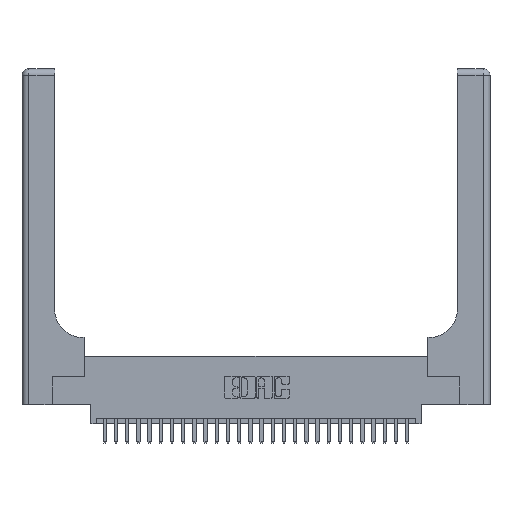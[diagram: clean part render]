
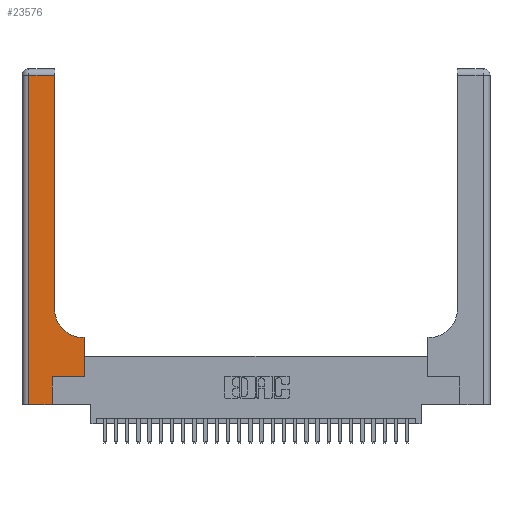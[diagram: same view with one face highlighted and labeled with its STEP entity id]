
A CAD part, top view. The second image highlights one B-rep face of the part: STEP entity #23576.
In plain terms, the highlighted planar face has unit normal (0, 0, 1).
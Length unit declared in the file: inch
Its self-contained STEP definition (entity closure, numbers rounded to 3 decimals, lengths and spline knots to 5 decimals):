
#175 = VERTEX_POINT ( 'NONE', #16787 ) ;
#555 = EDGE_CURVE ( 'NONE', #26798, #27050, #25872, .T. ) ;
#917 = ORIENTED_EDGE ( 'NONE', *, *, #14341, .T. ) ;
#1294 = VERTEX_POINT ( 'NONE', #22087 ) ;
#1426 = EDGE_CURVE ( 'NONE', #6271, #175, #9611, .T. ) ;
#1559 = AXIS2_PLACEMENT_3D ( 'NONE', #11578, #27400, #7145 ) ;
#2024 = CARTESIAN_POINT ( 'NONE',  ( 0.5415, 0.85, 0.37 ) ) ;
#2363 = LINE ( 'NONE', #13277, #22137 ) ;
#2943 = EDGE_LOOP ( 'NONE', ( #917, #24603, #6398, #16728, #15664, #22660, #19092, #27247, #21067 ) ) ;
#3328 = EDGE_CURVE ( 'NONE', #18350, #6271, #29008, .T. ) ;
#4276 = CARTESIAN_POINT ( 'NONE',  ( 0.269, 0.25, 0.37 ) ) ;
#4705 = CARTESIAN_POINT ( 'NONE',  ( 0.06, 0., 0.37 ) ) ;
#5241 = PLANE ( 'NONE',  #1559 ) ;
#5583 = DIRECTION ( 'NONE',  ( 0., -1., 0. ) ) ;
#5659 = CARTESIAN_POINT ( 'NONE',  ( 0., 2.94, 0.37 ) ) ;
#5894 = LINE ( 'NONE', #15029, #8032 ) ;
#6271 = VERTEX_POINT ( 'NONE', #4705 ) ;
#6398 = ORIENTED_EDGE ( 'NONE', *, *, #3328, .T. ) ;
#6661 = DIRECTION ( 'NONE',  ( 1., 0., 0. ) ) ;
#6663 = DIRECTION ( 'NONE',  ( 0., 0., -1. ) ) ;
#7078 = CARTESIAN_POINT ( 'NONE',  ( 0.06, 2.94, 0.37 ) ) ;
#7145 = DIRECTION ( 'NONE',  ( -1., 0., 0. ) ) ;
#8032 = VECTOR ( 'NONE', #22403, 39.37008 ) ;
#8461 = VERTEX_POINT ( 'NONE', #21993 ) ;
#8482 = VERTEX_POINT ( 'NONE', #11322 ) ;
#9213 = LINE ( 'NONE', #4276, #25836 ) ;
#9611 = LINE ( 'NONE', #24538, #20575 ) ;
#10365 = CARTESIAN_POINT ( 'NONE',  ( 0.06, 3., 0.37 ) ) ;
#11322 = CARTESIAN_POINT ( 'NONE',  ( 0.5585, 0.6, 0.37 ) ) ;
#11488 = CARTESIAN_POINT ( 'NONE',  ( 0.269, 0., 0.37 ) ) ;
#11578 = CARTESIAN_POINT ( 'NONE',  ( 0., 3., 0.37 ) ) ;
#13277 = CARTESIAN_POINT ( 'NONE',  ( 0.2915, 3., 0.37 ) ) ;
#14185 = LINE ( 'NONE', #5659, #25479 ) ;
#14341 = EDGE_CURVE ( 'NONE', #27050, #25663, #2363, .T. ) ;
#15029 = CARTESIAN_POINT ( 'NONE',  ( 0.2915, 0.6, 0.37 ) ) ;
#15216 = CARTESIAN_POINT ( 'NONE',  ( 0.2915, 0.85, 0.37 ) ) ;
#15538 = DIRECTION ( 'NONE',  ( 0., 1., 0. ) ) ;
#15664 = ORIENTED_EDGE ( 'NONE', *, *, #23378, .T. ) ;
#16692 = CARTESIAN_POINT ( 'NONE',  ( 0.5415, 0.6, 0.37 ) ) ;
#16728 = ORIENTED_EDGE ( 'NONE', *, *, #1426, .T. ) ;
#16787 = CARTESIAN_POINT ( 'NONE',  ( 0.269, 0., 0.37 ) ) ;
#17005 = CARTESIAN_POINT ( 'NONE',  ( 0.5585, 0.25, 0.37 ) ) ;
#18350 = VERTEX_POINT ( 'NONE', #7078 ) ;
#18672 = LINE ( 'NONE', #17005, #28979 ) ;
#19092 = ORIENTED_EDGE ( 'NONE', *, *, #28819, .T. ) ;
#19816 = VECTOR ( 'NONE', #5583, 39.37008 ) ;
#20575 = VECTOR ( 'NONE', #26343, 39.37008 ) ;
#20707 = VECTOR ( 'NONE', #22731, 39.37008 ) ;
#21067 = ORIENTED_EDGE ( 'NONE', *, *, #555, .T. ) ;
#21993 = CARTESIAN_POINT ( 'NONE',  ( 0.5585, 0.25, 0.37 ) ) ;
#22087 = CARTESIAN_POINT ( 'NONE',  ( 0.269, 0.25, 0.37 ) ) ;
#22137 = VECTOR ( 'NONE', #15538, 39.37008 ) ;
#22403 = DIRECTION ( 'NONE',  ( -1., 0., 0. ) ) ;
#22532 = DIRECTION ( 'NONE',  ( 1., 0., 0. ) ) ;
#22660 = ORIENTED_EDGE ( 'NONE', *, *, #27946, .T. ) ;
#22731 = DIRECTION ( 'NONE',  ( 0., 1., 0. ) ) ;
#22764 = EDGE_CURVE ( 'NONE', #8482, #26798, #5894, .T. ) ;
#23378 = EDGE_CURVE ( 'NONE', #175, #1294, #28884, .T. ) ;
#23576 = ADVANCED_FACE ( 'NONE', ( #27071 ), #5241, .F. ) ;
#23664 = CARTESIAN_POINT ( 'NONE',  ( 0.2915, 2.94, 0.37 ) ) ;
#24538 = CARTESIAN_POINT ( 'NONE',  ( 0., 0., 0.37 ) ) ;
#24603 = ORIENTED_EDGE ( 'NONE', *, *, #26480, .T. ) ;
#24835 = AXIS2_PLACEMENT_3D ( 'NONE', #2024, #6663, #22532 ) ;
#25479 = VECTOR ( 'NONE', #28396, 39.37008 ) ;
#25663 = VERTEX_POINT ( 'NONE', #23664 ) ;
#25836 = VECTOR ( 'NONE', #6661, 39.37008 ) ;
#25872 = CIRCLE ( 'NONE', #24835, 0.25 ) ;
#26343 = DIRECTION ( 'NONE',  ( 1., 0., 0. ) ) ;
#26480 = EDGE_CURVE ( 'NONE', #25663, #18350, #14185, .T. ) ;
#26798 = VERTEX_POINT ( 'NONE', #16692 ) ;
#27050 = VERTEX_POINT ( 'NONE', #15216 ) ;
#27071 = FACE_OUTER_BOUND ( 'NONE', #2943, .T. ) ;
#27247 = ORIENTED_EDGE ( 'NONE', *, *, #22764, .T. ) ;
#27400 = DIRECTION ( 'NONE',  ( 0., 0., -1. ) ) ;
#27946 = EDGE_CURVE ( 'NONE', #1294, #8461, #9213, .T. ) ;
#28266 = DIRECTION ( 'NONE',  ( 0., 1., 0. ) ) ;
#28396 = DIRECTION ( 'NONE',  ( -1., 0., 0. ) ) ;
#28819 = EDGE_CURVE ( 'NONE', #8461, #8482, #18672, .T. ) ;
#28884 = LINE ( 'NONE', #11488, #20707 ) ;
#28979 = VECTOR ( 'NONE', #28266, 39.37008 ) ;
#29008 = LINE ( 'NONE', #10365, #19816 ) ;
